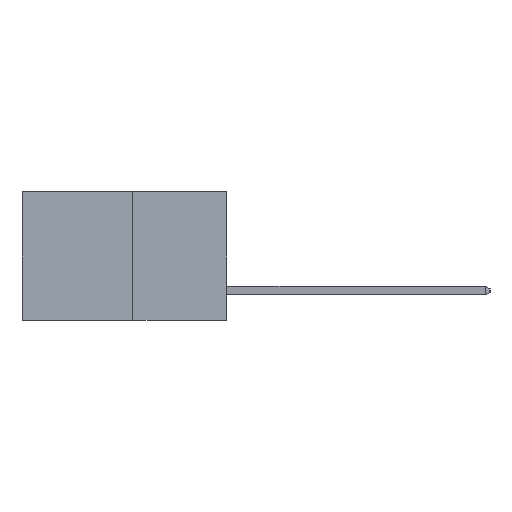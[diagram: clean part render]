
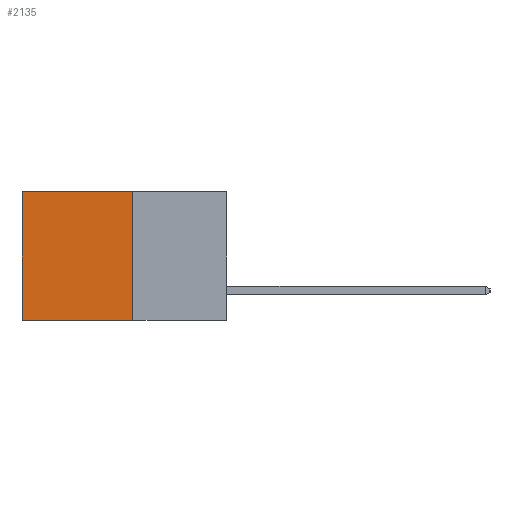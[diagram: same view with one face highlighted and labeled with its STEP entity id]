
A CAD part, left-side view. The second image highlights one B-rep face of the part: STEP entity #2135.
In plain terms, the highlighted planar face has unit normal (-1, 0, 0).
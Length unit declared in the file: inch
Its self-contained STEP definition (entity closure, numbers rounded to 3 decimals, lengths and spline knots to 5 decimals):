
#844 = DIRECTION ( 'NONE',  ( 0., 1., 0. ) ) ;
#868 = CARTESIAN_POINT ( 'NONE',  ( 0.277, 0.27, -0.37 ) ) ;
#1256 = LINE ( 'NONE', #868, #4955 ) ;
#1644 = ORIENTED_EDGE ( 'NONE', *, *, #7697, .T. ) ;
#1655 = ORIENTED_EDGE ( 'NONE', *, *, #4677, .F. ) ;
#1701 = ORIENTED_EDGE ( 'NONE', *, *, #5954, .F. ) ;
#1724 = ORIENTED_EDGE ( 'NONE', *, *, #6929, .T. ) ;
#1926 = VECTOR ( 'NONE', #6852, 39.37008 ) ;
#2000 = VERTEX_POINT ( 'NONE', #5857 ) ;
#2135 = ADVANCED_FACE ( 'NONE', ( #2378 ), #5908, .F. ) ;
#2167 = DIRECTION ( 'NONE',  ( 0., 1., 0. ) ) ;
#2285 = CARTESIAN_POINT ( 'NONE',  ( 0.277, 0.27, 0. ) ) ;
#2378 = FACE_OUTER_BOUND ( 'NONE', #6611, .T. ) ;
#3781 = VERTEX_POINT ( 'NONE', #5818 ) ;
#4162 = DIRECTION ( 'NONE',  ( 1., 0., 0. ) ) ;
#4677 = EDGE_CURVE ( 'NONE', #3781, #2000, #1256, .T. ) ;
#4955 = VECTOR ( 'NONE', #844, 39.37008 ) ;
#5026 = CARTESIAN_POINT ( 'NONE',  ( 0.277, 0.59, 0. ) ) ;
#5818 = CARTESIAN_POINT ( 'NONE',  ( 0.277, 0.27, -0.37 ) ) ;
#5857 = CARTESIAN_POINT ( 'NONE',  ( 0.277, 0.59, -0.37 ) ) ;
#5908 = PLANE ( 'NONE',  #8371 ) ;
#5954 = EDGE_CURVE ( 'NONE', #8885, #3781, #7552, .T. ) ;
#6119 = CARTESIAN_POINT ( 'NONE',  ( 0.277, 0.27, 0. ) ) ;
#6302 = VECTOR ( 'NONE', #2167, 39.37008 ) ;
#6398 = VERTEX_POINT ( 'NONE', #5026 ) ;
#6611 = EDGE_LOOP ( 'NONE', ( #1644, #1655, #1701, #1724 ) ) ;
#6776 = DIRECTION ( 'NONE',  ( 0., 0., -1. ) ) ;
#6852 = DIRECTION ( 'NONE',  ( 0., 0., -1. ) ) ;
#6858 = CARTESIAN_POINT ( 'NONE',  ( 0.277, 0.27, -0.37 ) ) ;
#6887 = CARTESIAN_POINT ( 'NONE',  ( 0.277, 0.27, -0.37 ) ) ;
#6929 = EDGE_CURVE ( 'NONE', #8885, #6398, #8051, .T. ) ;
#7137 = LINE ( 'NONE', #7476, #8765 ) ;
#7347 = DIRECTION ( 'NONE',  ( 0., 0., -1. ) ) ;
#7476 = CARTESIAN_POINT ( 'NONE',  ( 0.277, 0.59, -0.37 ) ) ;
#7552 = LINE ( 'NONE', #6858, #1926 ) ;
#7697 = EDGE_CURVE ( 'NONE', #6398, #2000, #7137, .T. ) ;
#8051 = LINE ( 'NONE', #2285, #6302 ) ;
#8371 = AXIS2_PLACEMENT_3D ( 'NONE', #6887, #4162, #6776 ) ;
#8765 = VECTOR ( 'NONE', #7347, 39.37008 ) ;
#8885 = VERTEX_POINT ( 'NONE', #6119 ) ;
